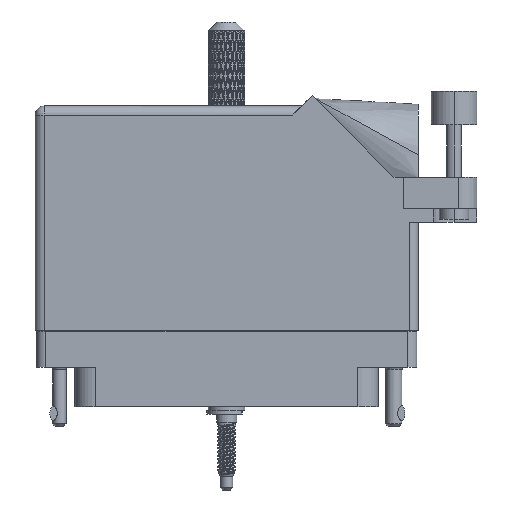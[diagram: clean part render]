
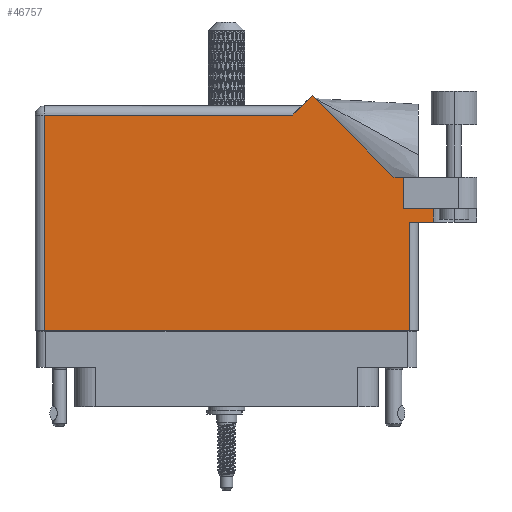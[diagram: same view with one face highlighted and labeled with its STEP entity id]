
A CAD part, front view. The second image highlights one B-rep face of the part: STEP entity #46757.
In plain terms, the highlighted face is planar.
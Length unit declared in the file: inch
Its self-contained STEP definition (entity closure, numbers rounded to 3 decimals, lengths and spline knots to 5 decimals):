
#2315 = EDGE_CURVE ( 'NONE', #71315, #119515, #76174, .T. ) ;
#2941 = CARTESIAN_POINT ( 'NONE',  ( -1.244, -0.1, 0.455 ) ) ;
#3338 = CARTESIAN_POINT ( 'NONE',  ( 1.244, -0.1, 0.455 ) ) ;
#6937 = ORIENTED_EDGE ( 'NONE', *, *, #88588, .F. ) ;
#7992 = VERTEX_POINT ( 'NONE', #116387 ) ;
#9087 = VERTEX_POINT ( 'NONE', #84211 ) ;
#10654 = LINE ( 'NONE', #40133, #108449 ) ;
#12863 = CARTESIAN_POINT ( 'NONE',  ( 1.14042, 0.944, 0.455 ) ) ;
#12949 = DIRECTION ( 'NONE',  ( 0., -1., 0. ) ) ;
#14617 = LINE ( 'NONE', #12863, #100665 ) ;
#14947 = EDGE_CURVE ( 'NONE', #112717, #7992, #121586, .T. ) ;
#16460 = CARTESIAN_POINT ( 'NONE',  ( -1.306, -0.1, 0.455 ) ) ;
#17767 = DIRECTION ( 'NONE',  ( -1., 0., 0. ) ) ;
#18228 = DIRECTION ( 'NONE',  ( 0., -1., 0. ) ) ;
#20421 = EDGE_CURVE ( 'NONE', #50403, #122648, #53022, .T. ) ;
#23783 = VECTOR ( 'NONE', #12949, 39.37008 ) ;
#24224 = VECTOR ( 'NONE', #114510, 39.37008 ) ;
#24382 = ORIENTED_EDGE ( 'NONE', *, *, #26053, .T. ) ;
#25188 = EDGE_CURVE ( 'NONE', #61961, #50403, #65702, .T. ) ;
#26053 = EDGE_CURVE ( 'NONE', #7992, #60535, #114539, .T. ) ;
#28558 = PLANE ( 'NONE',  #44693 ) ;
#31179 = LINE ( 'NONE', #111785, #48889 ) ;
#31794 = FACE_OUTER_BOUND ( 'NONE', #58400, .T. ) ;
#32495 = EDGE_CURVE ( 'NONE', #57363, #71315, #31179, .T. ) ;
#34318 = DIRECTION ( 'NONE',  ( 1., 0., 0. ) ) ;
#34350 = DIRECTION ( 'NONE',  ( -0.707, 0.707, 0. ) ) ;
#34432 = VECTOR ( 'NONE', #121206, 39.37008 ) ;
#35997 = CARTESIAN_POINT ( 'NONE',  ( 1.206, 0.731, 0.455 ) ) ;
#37271 = CARTESIAN_POINT ( 'NONE',  ( -1.244, -0.1, 0.455 ) ) ;
#37834 = ORIENTED_EDGE ( 'NONE', *, *, #76338, .T. ) ;
#39266 = EDGE_CURVE ( 'NONE', #112717, #79359, #10654, .T. ) ;
#40133 = CARTESIAN_POINT ( 'NONE',  ( 1.206, 0.731, 0.455 ) ) ;
#44243 = ORIENTED_EDGE ( 'NONE', *, *, #2315, .T. ) ;
#44693 = AXIS2_PLACEMENT_3D ( 'NONE', #103955, #56742, #57547 ) ;
#45035 = ORIENTED_EDGE ( 'NONE', *, *, #39266, .F. ) ;
#45507 = DIRECTION ( 'NONE',  ( 0., 1., 0. ) ) ;
#45981 = VECTOR ( 'NONE', #45507, 39.37008 ) ;
#46757 = ADVANCED_FACE ( 'NONE', ( #31794 ), #28558, .F. ) ;
#48889 = VECTOR ( 'NONE', #54172, 39.37008 ) ;
#49780 = CARTESIAN_POINT ( 'NONE',  ( 0.451, 1.368, 0.455 ) ) ;
#50185 = CARTESIAN_POINT ( 'NONE',  ( 1.4075, 1.06177, 0.455 ) ) ;
#50403 = VERTEX_POINT ( 'NONE', #91985 ) ;
#50597 = ORIENTED_EDGE ( 'NONE', *, *, #14947, .T. ) ;
#50608 = CARTESIAN_POINT ( 'NONE',  ( 1.306, 0.637, 0.455 ) ) ;
#53022 = LINE ( 'NONE', #37271, #72324 ) ;
#54172 = DIRECTION ( 'NONE',  ( 0., 1., 0. ) ) ;
#55828 = CARTESIAN_POINT ( 'NONE',  ( 1.206, 0.731, 0.455 ) ) ;
#56742 = DIRECTION ( 'NONE',  ( 0., 0., -1. ) ) ;
#57363 = VERTEX_POINT ( 'NONE', #3338 ) ;
#57547 = DIRECTION ( 'NONE',  ( -1., 0., 0. ) ) ;
#58400 = EDGE_LOOP ( 'NONE', ( #71115, #97244, #44243, #6937, #45035, #50597, #24382, #102755, #37834, #85409, #112661 ) ) ;
#58908 = CARTESIAN_POINT ( 'NONE',  ( 0.513, 1.43, 0.455 ) ) ;
#60535 = VERTEX_POINT ( 'NONE', #75734 ) ;
#61169 = VECTOR ( 'NONE', #17767, 39.37008 ) ;
#61961 = VERTEX_POINT ( 'NONE', #49780 ) ;
#65702 = LINE ( 'NONE', #86707, #24224 ) ;
#71115 = ORIENTED_EDGE ( 'NONE', *, *, #119486, .T. ) ;
#71315 = VERTEX_POINT ( 'NONE', #79496 ) ;
#72324 = VECTOR ( 'NONE', #18228, 39.37008 ) ;
#73182 = VECTOR ( 'NONE', #34318, 39.37008 ) ;
#75734 = CARTESIAN_POINT ( 'NONE',  ( 1.14042, 0.944, 0.455 ) ) ;
#76174 = LINE ( 'NONE', #50608, #73182 ) ;
#76338 = EDGE_CURVE ( 'NONE', #9087, #61961, #83341, .T. ) ;
#79359 = VERTEX_POINT ( 'NONE', #85556 ) ;
#79496 = CARTESIAN_POINT ( 'NONE',  ( 1.244, 0.637, 0.455 ) ) ;
#83341 = LINE ( 'NONE', #58908, #114469 ) ;
#84211 = CARTESIAN_POINT ( 'NONE',  ( 0.58371, 1.50071, 0.455 ) ) ;
#85409 = ORIENTED_EDGE ( 'NONE', *, *, #25188, .T. ) ;
#85556 = CARTESIAN_POINT ( 'NONE',  ( 1.4075, 0.731, 0.455 ) ) ;
#86707 = CARTESIAN_POINT ( 'NONE',  ( -1.306, 1.368, 0.455 ) ) ;
#88588 = EDGE_CURVE ( 'NONE', #79359, #119515, #108248, .T. ) ;
#89213 = LINE ( 'NONE', #16460, #34432 ) ;
#91985 = CARTESIAN_POINT ( 'NONE',  ( -1.244, 1.368, 0.455 ) ) ;
#93082 = CARTESIAN_POINT ( 'NONE',  ( 1.4075, 0.637, 0.455 ) ) ;
#93594 = CARTESIAN_POINT ( 'NONE',  ( 1.706, 0.944, 0.455 ) ) ;
#97244 = ORIENTED_EDGE ( 'NONE', *, *, #32495, .T. ) ;
#99872 = EDGE_CURVE ( 'NONE', #60535, #9087, #14617, .T. ) ;
#100665 = VECTOR ( 'NONE', #34350, 39.37008 ) ;
#102755 = ORIENTED_EDGE ( 'NONE', *, *, #99872, .T. ) ;
#103955 = CARTESIAN_POINT ( 'NONE',  ( -1.306, 1.43, 0.455 ) ) ;
#106423 = DIRECTION ( 'NONE',  ( 1., 0., 0. ) ) ;
#108248 = LINE ( 'NONE', #50185, #23783 ) ;
#108449 = VECTOR ( 'NONE', #106423, 39.37008 ) ;
#111785 = CARTESIAN_POINT ( 'NONE',  ( 1.244, 0.637, 0.455 ) ) ;
#112661 = ORIENTED_EDGE ( 'NONE', *, *, #20421, .T. ) ;
#112717 = VERTEX_POINT ( 'NONE', #55828 ) ;
#114411 = DIRECTION ( 'NONE',  ( -0.707, -0.707, 0. ) ) ;
#114469 = VECTOR ( 'NONE', #114411, 39.37008 ) ;
#114510 = DIRECTION ( 'NONE',  ( -1., 0., 0. ) ) ;
#114539 = LINE ( 'NONE', #93594, #61169 ) ;
#116387 = CARTESIAN_POINT ( 'NONE',  ( 1.206, 0.944, 0.455 ) ) ;
#119486 = EDGE_CURVE ( 'NONE', #122648, #57363, #89213, .T. ) ;
#119515 = VERTEX_POINT ( 'NONE', #93082 ) ;
#121206 = DIRECTION ( 'NONE',  ( 1., 0., 0. ) ) ;
#121586 = LINE ( 'NONE', #35997, #45981 ) ;
#122648 = VERTEX_POINT ( 'NONE', #2941 ) ;
